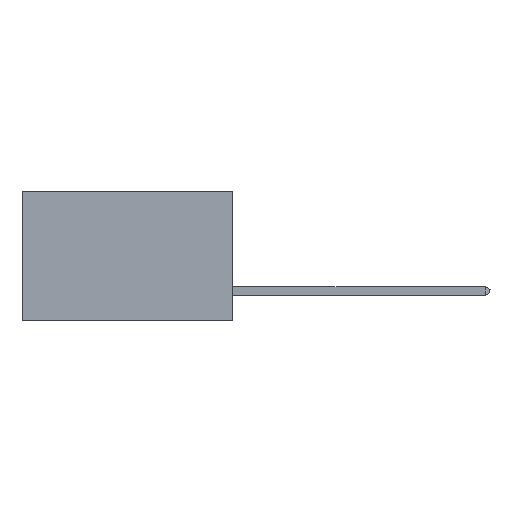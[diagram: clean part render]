
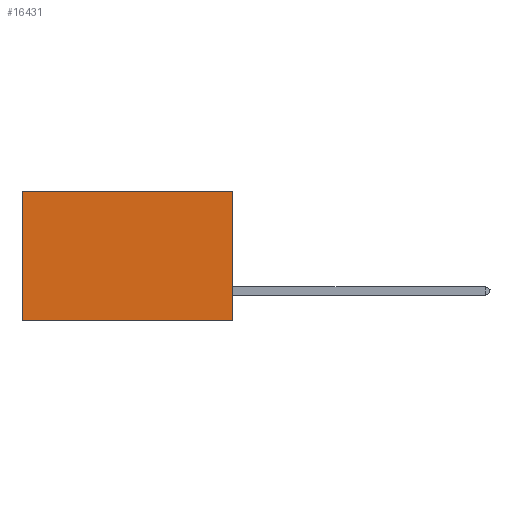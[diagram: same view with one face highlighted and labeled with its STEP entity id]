
A CAD part, left-side view. The second image highlights one B-rep face of the part: STEP entity #16431.
In plain terms, the highlighted planar face has unit normal (-1, 0, 0).
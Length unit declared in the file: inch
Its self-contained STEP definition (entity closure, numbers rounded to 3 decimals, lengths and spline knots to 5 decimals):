
#178 = EDGE_CURVE ( 'NONE', #20949, #18032, #8802, .T. ) ;
#1280 = EDGE_CURVE ( 'NONE', #15463, #13844, #6597, .T. ) ;
#3462 = PLANE ( 'NONE',  #20404 ) ;
#3856 = DIRECTION ( 'NONE',  ( 0., 0., -1. ) ) ;
#4295 = DIRECTION ( 'NONE',  ( 1., 0., 0. ) ) ;
#4672 = EDGE_CURVE ( 'NONE', #18032, #13844, #24341, .T. ) ;
#5558 = VECTOR ( 'NONE', #28239, 39.37008 ) ;
#5977 = ORIENTED_EDGE ( 'NONE', *, *, #31665, .T. ) ;
#6571 = EDGE_LOOP ( 'NONE', ( #39752, #13253, #18520, #5977 ) ) ;
#6597 = LINE ( 'NONE', #14761, #5558 ) ;
#8517 = DIRECTION ( 'NONE',  ( 0., 1., 0. ) ) ;
#8802 = LINE ( 'NONE', #40241, #34690 ) ;
#13253 = ORIENTED_EDGE ( 'NONE', *, *, #4672, .F. ) ;
#13844 = VERTEX_POINT ( 'NONE', #27410 ) ;
#14761 = CARTESIAN_POINT ( 'NONE',  ( 0.2875, 0.6, 0. ) ) ;
#15463 = VERTEX_POINT ( 'NONE', #41952 ) ;
#16431 = ADVANCED_FACE ( 'NONE', ( #36807 ), #3462, .F. ) ;
#17642 = VECTOR ( 'NONE', #22394, 39.37008 ) ;
#18032 = VERTEX_POINT ( 'NONE', #18523 ) ;
#18520 = ORIENTED_EDGE ( 'NONE', *, *, #178, .F. ) ;
#18523 = CARTESIAN_POINT ( 'NONE',  ( 0.2875, 0., -0.37 ) ) ;
#19758 = CARTESIAN_POINT ( 'NONE',  ( 0.2875, 0., 0. ) ) ;
#20404 = AXIS2_PLACEMENT_3D ( 'NONE', #37018, #4295, #3856 ) ;
#20949 = VERTEX_POINT ( 'NONE', #30747 ) ;
#22394 = DIRECTION ( 'NONE',  ( 0., 1., 0. ) ) ;
#23824 = DIRECTION ( 'NONE',  ( 0., 0., -1. ) ) ;
#24341 = LINE ( 'NONE', #28068, #17642 ) ;
#27410 = CARTESIAN_POINT ( 'NONE',  ( 0.2875, 0.6, -0.37 ) ) ;
#28068 = CARTESIAN_POINT ( 'NONE',  ( 0.2875, 0., -0.37 ) ) ;
#28239 = DIRECTION ( 'NONE',  ( 0., 0., -1. ) ) ;
#30747 = CARTESIAN_POINT ( 'NONE',  ( 0.2875, 0., 0. ) ) ;
#31665 = EDGE_CURVE ( 'NONE', #20949, #15463, #35713, .T. ) ;
#34690 = VECTOR ( 'NONE', #23824, 39.37008 ) ;
#35167 = VECTOR ( 'NONE', #8517, 39.37008 ) ;
#35713 = LINE ( 'NONE', #19758, #35167 ) ;
#36807 = FACE_OUTER_BOUND ( 'NONE', #6571, .T. ) ;
#37018 = CARTESIAN_POINT ( 'NONE',  ( 0.2875, 0., 0. ) ) ;
#39752 = ORIENTED_EDGE ( 'NONE', *, *, #1280, .T. ) ;
#40241 = CARTESIAN_POINT ( 'NONE',  ( 0.2875, 0., 0. ) ) ;
#41952 = CARTESIAN_POINT ( 'NONE',  ( 0.2875, 0.6, 0. ) ) ;
